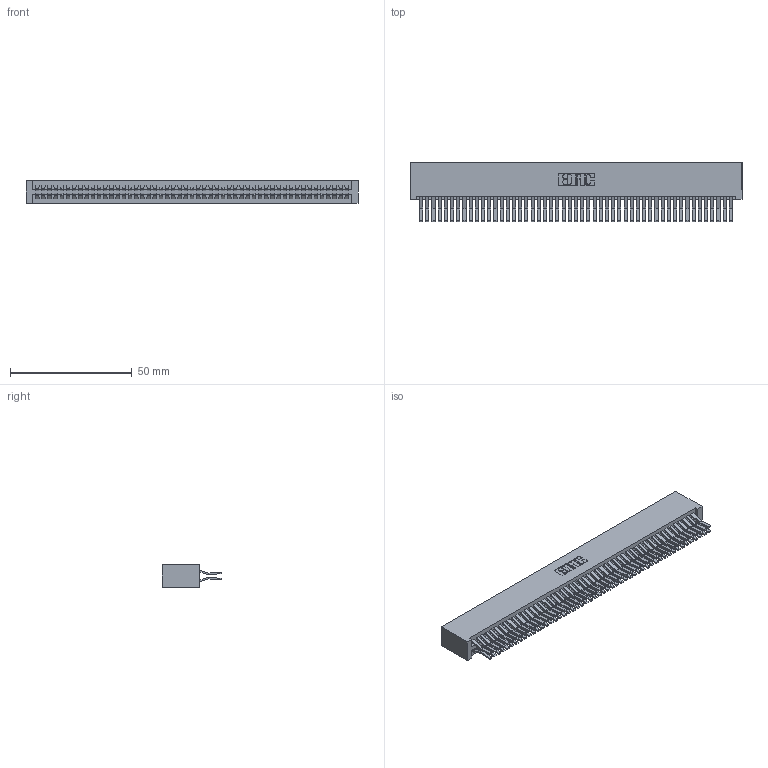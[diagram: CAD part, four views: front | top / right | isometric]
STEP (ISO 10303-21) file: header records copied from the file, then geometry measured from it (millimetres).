
FILE_DESCRIPTION (( 'STEP AP203' ), '1' );
FILE_NAME ('395-102-560-201.STEP', '2019-10-26T19:39:37', ( '' ), ( '' ), 'SwSTEP 2.0', 'SolidWorks 2016', '' );
FILE_SCHEMA (( 'CONFIG_CONTROL_DESIGN' ));
Length unit declared in the file: inch
Products named in the file (3): 345 Part_No Mounting Lugs; 345-292-001_560 Tail; 395-102-560-201
Assembly tree (103 placements, depth 2):
  395-102-560-201
    345 Part_No Mounting Lugs
    345-292-001_560 Tail  x102
Bounding box: 136.14 x 24.45 x 9.4 mm (x, y, z)
Volume: 14593.2 mm3; surface area: 23768.3 mm2
Topology: 103 solids, 103 shells, 5422 faces, 16127 edges, 10614 vertices
Faces by surface type: plane 3442, cylinder 1980
Entity records: 38615 total; most frequent: CARTESIAN_POINT 6464, ORIENTED_EDGE 6398, DIRECTION 5687, EDGE_CURVE 3199, LINE 2867, VECTOR 2867, VERTEX_POINT 2130, AXIS2_PLACEMENT_3D 1410
